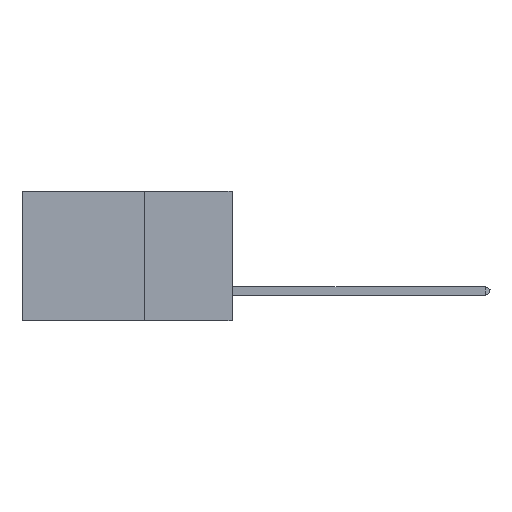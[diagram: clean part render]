
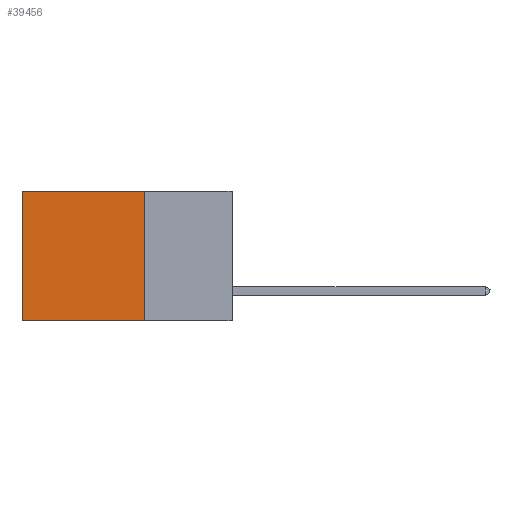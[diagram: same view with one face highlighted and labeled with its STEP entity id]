
A CAD part, left-side view. The second image highlights one B-rep face of the part: STEP entity #39456.
In plain terms, the highlighted planar face has unit normal (-1, 0, 0).
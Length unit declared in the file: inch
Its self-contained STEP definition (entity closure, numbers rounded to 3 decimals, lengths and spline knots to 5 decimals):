
#488 = CARTESIAN_POINT ( 'NONE',  ( 0.2875, 0.25, -0.37 ) ) ;
#971 = CARTESIAN_POINT ( 'NONE',  ( 0.2875, 0.6, -0.37 ) ) ;
#1425 = FACE_OUTER_BOUND ( 'NONE', #17430, .T. ) ;
#1777 = VERTEX_POINT ( 'NONE', #32209 ) ;
#3431 = ORIENTED_EDGE ( 'NONE', *, *, #29606, .F. ) ;
#3924 = CARTESIAN_POINT ( 'NONE',  ( 0.2875, 0.6, 0. ) ) ;
#4771 = VERTEX_POINT ( 'NONE', #7927 ) ;
#5879 = PLANE ( 'NONE',  #42749 ) ;
#7654 = DIRECTION ( 'NONE',  ( 0., 1., 0. ) ) ;
#7927 = CARTESIAN_POINT ( 'NONE',  ( 0.2875, 0.25, -0.37 ) ) ;
#8638 = CARTESIAN_POINT ( 'NONE',  ( 0.2875, 0.25, 0. ) ) ;
#9073 = VECTOR ( 'NONE', #7654, 39.37008 ) ;
#9619 = VERTEX_POINT ( 'NONE', #8638 ) ;
#10937 = CARTESIAN_POINT ( 'NONE',  ( 0.2875, 0.25, 0. ) ) ;
#12890 = EDGE_CURVE ( 'NONE', #9619, #4771, #40004, .T. ) ;
#13337 = ORIENTED_EDGE ( 'NONE', *, *, #15550, .T. ) ;
#14387 = VECTOR ( 'NONE', #23787, 39.37008 ) ;
#14690 = VECTOR ( 'NONE', #24186, 39.37008 ) ;
#15467 = LINE ( 'NONE', #488, #14387 ) ;
#15550 = EDGE_CURVE ( 'NONE', #9619, #1777, #15830, .T. ) ;
#15795 = EDGE_CURVE ( 'NONE', #1777, #19818, #28894, .T. ) ;
#15830 = LINE ( 'NONE', #10937, #9073 ) ;
#17430 = EDGE_LOOP ( 'NONE', ( #20784, #3431, #30179, #13337 ) ) ;
#19818 = VERTEX_POINT ( 'NONE', #971 ) ;
#20784 = ORIENTED_EDGE ( 'NONE', *, *, #15795, .T. ) ;
#23787 = DIRECTION ( 'NONE',  ( 0., 1., 0. ) ) ;
#24186 = DIRECTION ( 'NONE',  ( 0., 0., -1. ) ) ;
#24331 = DIRECTION ( 'NONE',  ( 0., 0., -1. ) ) ;
#28894 = LINE ( 'NONE', #3924, #14690 ) ;
#29070 = CARTESIAN_POINT ( 'NONE',  ( 0.2875, 0.25, 0. ) ) ;
#29606 = EDGE_CURVE ( 'NONE', #4771, #19818, #15467, .T. ) ;
#30179 = ORIENTED_EDGE ( 'NONE', *, *, #12890, .F. ) ;
#32209 = CARTESIAN_POINT ( 'NONE',  ( 0.2875, 0.6, 0. ) ) ;
#32645 = DIRECTION ( 'NONE',  ( 1., 0., 0. ) ) ;
#32844 = VECTOR ( 'NONE', #24331, 39.37008 ) ;
#35625 = CARTESIAN_POINT ( 'NONE',  ( 0.2875, 0.25, 0. ) ) ;
#39456 = ADVANCED_FACE ( 'NONE', ( #1425 ), #5879, .F. ) ;
#40004 = LINE ( 'NONE', #35625, #32844 ) ;
#42464 = DIRECTION ( 'NONE',  ( 0., 0., -1. ) ) ;
#42749 = AXIS2_PLACEMENT_3D ( 'NONE', #29070, #32645, #42464 ) ;
